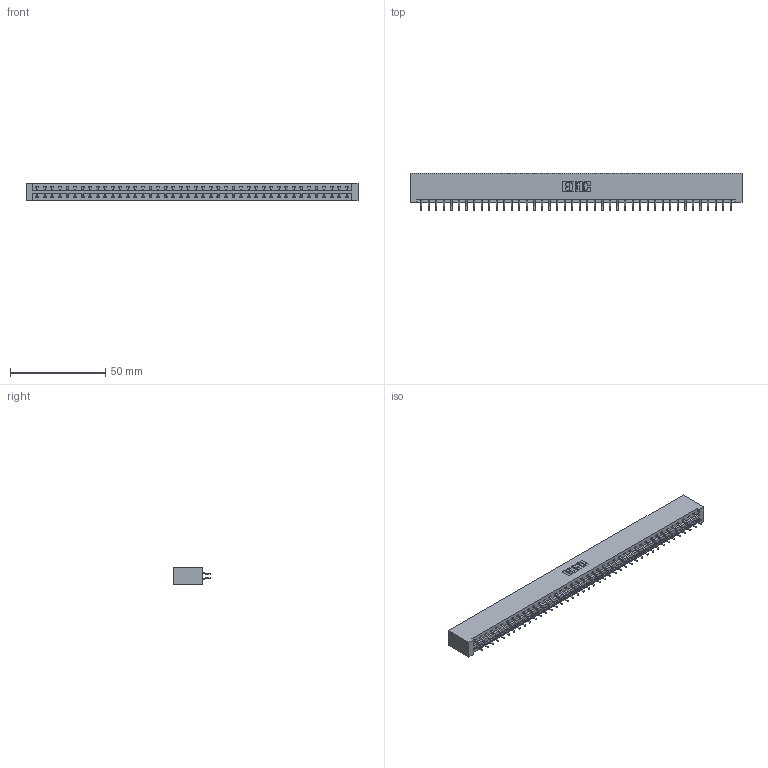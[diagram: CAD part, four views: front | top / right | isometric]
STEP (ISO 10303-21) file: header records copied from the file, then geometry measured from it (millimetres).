
FILE_DESCRIPTION (( 'STEP AP203' ), '1' );
FILE_NAME ('337-084-556-201.STEP', '2019-10-10T14:17:00', ( '' ), ( '' ), 'SwSTEP 2.0', 'SolidWorks 2016', '' );
FILE_SCHEMA (( 'CONFIG_CONTROL_DESIGN' ));
Length unit declared in the file: inch
Products named in the file (3): 337-084-556-201; 337 Part_No Mounting Lugs; 345-292-001_556 Tail
Assembly tree (85 placements, depth 2):
  337-084-556-201
    337 Part_No Mounting Lugs
    345-292-001_556 Tail  x84
Bounding box: 174.29 x 19.57 x 9.4 mm (x, y, z)
Volume: 19126 mm3; surface area: 21589.4 mm2
Topology: 85 solids, 85 shells, 5146 faces, 15323 edges, 10102 vertices
Faces by surface type: plane 3594, cylinder 1552
Entity records: 32507 total; most frequent: CARTESIAN_POINT 5490, ORIENTED_EDGE 5414, DIRECTION 4651, EDGE_CURVE 2707, VECTOR 2579, LINE 2579, VERTEX_POINT 1802, AXIS2_PLACEMENT_3D 1036
